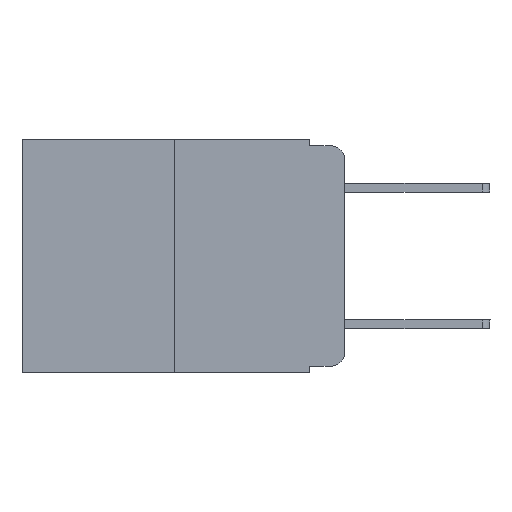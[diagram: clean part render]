
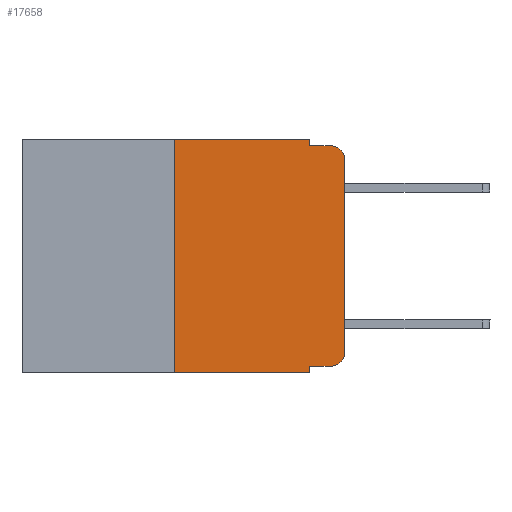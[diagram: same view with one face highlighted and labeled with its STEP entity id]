
A CAD part, left-side view. The second image highlights one B-rep face of the part: STEP entity #17658.
In plain terms, the highlighted planar face has unit normal (-1, 0, 0).
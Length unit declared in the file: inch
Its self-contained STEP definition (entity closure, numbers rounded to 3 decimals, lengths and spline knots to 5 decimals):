
#18 = CARTESIAN_POINT ( 'NONE',  ( 0., 0.25, 0. ) ) ;
#106 = DIRECTION ( 'NONE',  ( 0., -1., 0. ) ) ;
#449 = DIRECTION ( 'NONE',  ( 0., 0., 1. ) ) ;
#695 = VERTEX_POINT ( 'NONE', #19632 ) ;
#701 = EDGE_CURVE ( 'NONE', #8404, #695, #15017, .T. ) ;
#876 = LINE ( 'NONE', #18, #18512 ) ;
#1515 = ORIENTED_EDGE ( 'NONE', *, *, #701, .F. ) ;
#1518 = CIRCLE ( 'NONE', #4168, 0.02 ) ;
#1728 = VECTOR ( 'NONE', #13187, 39.37008 ) ;
#1753 = CARTESIAN_POINT ( 'NONE',  ( 0., 0.051, -0.343 ) ) ;
#1773 = CARTESIAN_POINT ( 'NONE',  ( 0., 0.473, 0. ) ) ;
#2071 = CARTESIAN_POINT ( 'NONE',  ( 0., 0., 0. ) ) ;
#2356 = CARTESIAN_POINT ( 'NONE',  ( 0., 0.25, -0.343 ) ) ;
#2881 = ORIENTED_EDGE ( 'NONE', *, *, #4442, .T. ) ;
#2959 = VERTEX_POINT ( 'NONE', #2356 ) ;
#3090 = AXIS2_PLACEMENT_3D ( 'NONE', #1773, #5134, #16257 ) ;
#3654 = VECTOR ( 'NONE', #106, 39.37008 ) ;
#3930 = VERTEX_POINT ( 'NONE', #3971 ) ;
#3971 = CARTESIAN_POINT ( 'NONE',  ( 0., 0., -0.03 ) ) ;
#4168 = AXIS2_PLACEMENT_3D ( 'NONE', #16617, #8446, #19725 ) ;
#4236 = FACE_OUTER_BOUND ( 'NONE', #15066, .T. ) ;
#4442 = EDGE_CURVE ( 'NONE', #8066, #3930, #16764, .T. ) ;
#4905 = CARTESIAN_POINT ( 'NONE',  ( 0., 0.25, 0. ) ) ;
#4939 = VECTOR ( 'NONE', #14306, 39.37008 ) ;
#5134 = DIRECTION ( 'NONE',  ( 1., 0., 0. ) ) ;
#5310 = DIRECTION ( 'NONE',  ( 0., -1., 0. ) ) ;
#5730 = VECTOR ( 'NONE', #14315, 39.37008 ) ;
#5994 = CARTESIAN_POINT ( 'NONE',  ( 0., 0., -0.313 ) ) ;
#5997 = LINE ( 'NONE', #12623, #4939 ) ;
#6203 = VERTEX_POINT ( 'NONE', #14804 ) ;
#6615 = VERTEX_POINT ( 'NONE', #1753 ) ;
#6929 = CARTESIAN_POINT ( 'NONE',  ( 0., 0.473, -0.343 ) ) ;
#6976 = ORIENTED_EDGE ( 'NONE', *, *, #15617, .F. ) ;
#7280 = LINE ( 'NONE', #20753, #5730 ) ;
#7635 = VERTEX_POINT ( 'NONE', #9613 ) ;
#8066 = VERTEX_POINT ( 'NONE', #5994 ) ;
#8404 = VERTEX_POINT ( 'NONE', #10221 ) ;
#8446 = DIRECTION ( 'NONE',  ( -1., 0., 0. ) ) ;
#8498 = EDGE_CURVE ( 'NONE', #9628, #8066, #1518, .T. ) ;
#8740 = VECTOR ( 'NONE', #5310, 39.37008 ) ;
#9115 = ORIENTED_EDGE ( 'NONE', *, *, #16646, .T. ) ;
#9387 = EDGE_CURVE ( 'NONE', #7635, #6615, #7280, .T. ) ;
#9613 = CARTESIAN_POINT ( 'NONE',  ( 0., 0.051, -0.333 ) ) ;
#9628 = VERTEX_POINT ( 'NONE', #19002 ) ;
#9837 = ORIENTED_EDGE ( 'NONE', *, *, #9387, .F. ) ;
#9983 = CARTESIAN_POINT ( 'NONE',  ( 0., 0.051, 0. ) ) ;
#9985 = ORIENTED_EDGE ( 'NONE', *, *, #11540, .F. ) ;
#10221 = CARTESIAN_POINT ( 'NONE',  ( 0., 0.051, -0.01 ) ) ;
#10286 = EDGE_CURVE ( 'NONE', #2959, #6615, #15759, .T. ) ;
#10360 = ORIENTED_EDGE ( 'NONE', *, *, #13781, .T. ) ;
#10716 = ORIENTED_EDGE ( 'NONE', *, *, #8498, .T. ) ;
#11254 = LINE ( 'NONE', #19199, #3654 ) ;
#11280 = ORIENTED_EDGE ( 'NONE', *, *, #10286, .T. ) ;
#11540 = EDGE_CURVE ( 'NONE', #14945, #6203, #11254, .T. ) ;
#11881 = DIRECTION ( 'NONE',  ( 0., 0., -1. ) ) ;
#12089 = CARTESIAN_POINT ( 'NONE',  ( 0., 0.02, -0.03 ) ) ;
#12403 = EDGE_CURVE ( 'NONE', #2959, #14945, #876, .T. ) ;
#12567 = LINE ( 'NONE', #9983, #1728 ) ;
#12623 = CARTESIAN_POINT ( 'NONE',  ( 0., 0.051, -0.333 ) ) ;
#13187 = DIRECTION ( 'NONE',  ( 0., 0., -1. ) ) ;
#13781 = EDGE_CURVE ( 'NONE', #3930, #695, #16689, .T. ) ;
#14306 = DIRECTION ( 'NONE',  ( 0., -1., 0. ) ) ;
#14315 = DIRECTION ( 'NONE',  ( 0., 0., -1. ) ) ;
#14757 = VECTOR ( 'NONE', #14792, 39.37008 ) ;
#14792 = DIRECTION ( 'NONE',  ( 0., -1., 0. ) ) ;
#14804 = CARTESIAN_POINT ( 'NONE',  ( 0., 0.051, 0. ) ) ;
#14945 = VERTEX_POINT ( 'NONE', #4905 ) ;
#14951 = CARTESIAN_POINT ( 'NONE',  ( 0., 0.051, -0.01 ) ) ;
#15017 = LINE ( 'NONE', #14951, #8740 ) ;
#15066 = EDGE_LOOP ( 'NONE', ( #2881, #10360, #1515, #6976, #9985, #19339, #11280, #9837, #9115, #10716 ) ) ;
#15617 = EDGE_CURVE ( 'NONE', #6203, #8404, #12567, .T. ) ;
#15759 = LINE ( 'NONE', #6929, #14757 ) ;
#15849 = DIRECTION ( 'NONE',  ( 0., 0., 1. ) ) ;
#16257 = DIRECTION ( 'NONE',  ( 0., 0., -1. ) ) ;
#16617 = CARTESIAN_POINT ( 'NONE',  ( 0., 0.02, -0.313 ) ) ;
#16646 = EDGE_CURVE ( 'NONE', #7635, #9628, #5997, .T. ) ;
#16689 = CIRCLE ( 'NONE', #17081, 0.02 ) ;
#16764 = LINE ( 'NONE', #2071, #18299 ) ;
#16793 = DIRECTION ( 'NONE',  ( -1., 0., 0. ) ) ;
#17081 = AXIS2_PLACEMENT_3D ( 'NONE', #12089, #16793, #11881 ) ;
#17658 = ADVANCED_FACE ( 'NONE', ( #4236 ), #19381, .F. ) ;
#18299 = VECTOR ( 'NONE', #449, 39.37008 ) ;
#18512 = VECTOR ( 'NONE', #15849, 39.37008 ) ;
#19002 = CARTESIAN_POINT ( 'NONE',  ( 0., 0.02, -0.333 ) ) ;
#19199 = CARTESIAN_POINT ( 'NONE',  ( 0., 0.473, 0. ) ) ;
#19339 = ORIENTED_EDGE ( 'NONE', *, *, #12403, .F. ) ;
#19381 = PLANE ( 'NONE',  #3090 ) ;
#19632 = CARTESIAN_POINT ( 'NONE',  ( 0., 0.02, -0.01 ) ) ;
#19725 = DIRECTION ( 'NONE',  ( 0., 0., -1. ) ) ;
#20753 = CARTESIAN_POINT ( 'NONE',  ( 0., 0.051, 0. ) ) ;
